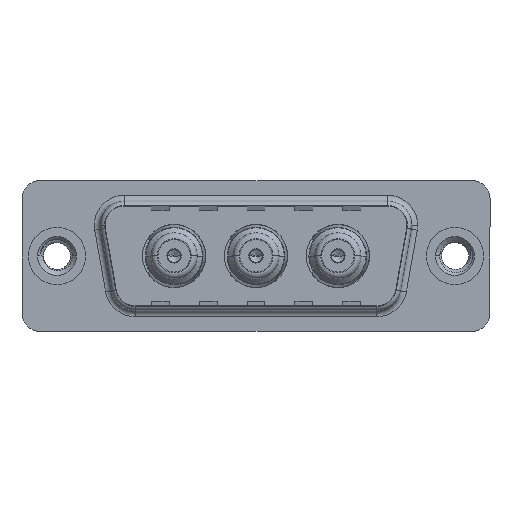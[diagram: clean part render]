
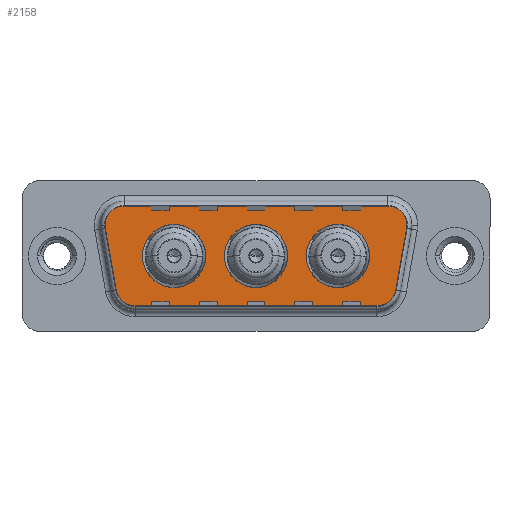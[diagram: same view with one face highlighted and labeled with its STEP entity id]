
A CAD part, top view. The second image highlights one B-rep face of the part: STEP entity #2158.
In plain terms, the highlighted planar face has unit normal (0, 0, 1).
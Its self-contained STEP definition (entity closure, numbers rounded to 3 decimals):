
#181 = CIRCLE ( 'NONE', #14283, 2.65 ) ;
#232 = DIRECTION ( 'NONE',  ( 1., 0., 0. ) ) ;
#323 = CARTESIAN_POINT ( 'NONE',  ( 3.441, 2.553, 0. ) ) ;
#436 = EDGE_LOOP ( 'NONE', ( #1682, #2005 ) ) ;
#500 = EDGE_CURVE ( 'NONE', #17174, #4676, #1837, .T. ) ;
#673 = CARTESIAN_POINT ( 'NONE',  ( 28.836, -3.247, 0. ) ) ;
#916 = DIRECTION ( 'NONE',  ( 1., 0., 0. ) ) ;
#1031 = VERTEX_POINT ( 'NONE', #10401 ) ;
#1154 = AXIS2_PLACEMENT_3D ( 'NONE', #15746, #4045, #232 ) ;
#1682 = ORIENTED_EDGE ( 'NONE', *, *, #6359, .F. ) ;
#1809 = PLANE ( 'NONE',  #12351 ) ;
#1837 = LINE ( 'NONE', #5329, #13462 ) ;
#1903 = CIRCLE ( 'NONE', #2619, 2.65 ) ;
#1958 = DIRECTION ( 'NONE',  ( 1., 0., 0. ) ) ;
#2002 = AXIS2_PLACEMENT_3D ( 'NONE', #4181, #14785, #5699 ) ;
#2005 = ORIENTED_EDGE ( 'NONE', *, *, #2195, .F. ) ;
#2093 = DIRECTION ( 'NONE',  ( -1., 0., 0. ) ) ;
#2158 = ADVANCED_FACE ( 'NONE', ( #16734, #5149, #18129, #12742 ), #1809, .T. ) ;
#2195 = EDGE_CURVE ( 'NONE', #3251, #8735, #4196, .T. ) ;
#2500 = VERTEX_POINT ( 'NONE', #8867 ) ;
#2619 = AXIS2_PLACEMENT_3D ( 'NONE', #13591, #13808, #13867 ) ;
#2841 = DIRECTION ( 'NONE',  ( 1., 0., 0. ) ) ;
#2946 = EDGE_CURVE ( 'NONE', #10367, #4493, #3212, .T. ) ;
#3025 = CARTESIAN_POINT ( 'NONE',  ( 16.65, 0., 0. ) ) ;
#3212 = CIRCLE ( 'NONE', #7172, 2.65 ) ;
#3251 = VERTEX_POINT ( 'NONE', #14914 ) ;
#3342 = CIRCLE ( 'NONE', #14150, 2. ) ;
#3473 = EDGE_CURVE ( 'NONE', #14745, #5964, #15758, .T. ) ;
#3595 = EDGE_CURVE ( 'NONE', #9859, #11575, #17843, .T. ) ;
#3685 = VECTOR ( 'NONE', #16691, 1000. ) ;
#3847 = AXIS2_PLACEMENT_3D ( 'NONE', #8420, #18898, #9929 ) ;
#4045 = DIRECTION ( 'NONE',  ( 0., 0., 1. ) ) ;
#4118 = CARTESIAN_POINT ( 'NONE',  ( 26.866, -4.9, 0. ) ) ;
#4178 = CIRCLE ( 'NONE', #9466, 2. ) ;
#4181 = CARTESIAN_POINT ( 'NONE',  ( 5.411, 2.9, 0. ) ) ;
#4196 = CIRCLE ( 'NONE', #14377, 2.65 ) ;
#4300 = DIRECTION ( 'NONE',  ( 0.174, 0.985, 0. ) ) ;
#4339 = CARTESIAN_POINT ( 'NONE',  ( 6.434, -4.9, 0. ) ) ;
#4355 = EDGE_CURVE ( 'NONE', #4493, #10367, #15504, .T. ) ;
#4493 = VERTEX_POINT ( 'NONE', #9935 ) ;
#4676 = VERTEX_POINT ( 'NONE', #7659 ) ;
#4897 = VERTEX_POINT ( 'NONE', #4118 ) ;
#4936 = VECTOR ( 'NONE', #1958, 1000. ) ;
#5143 = ORIENTED_EDGE ( 'NONE', *, *, #4355, .F. ) ;
#5149 = FACE_BOUND ( 'NONE', #9118, .T. ) ;
#5166 = CARTESIAN_POINT ( 'NONE',  ( 19.3, 0., 0. ) ) ;
#5329 = CARTESIAN_POINT ( 'NONE',  ( 3.441, 2.553, 0. ) ) ;
#5501 = EDGE_CURVE ( 'NONE', #10274, #1031, #181, .T. ) ;
#5699 = DIRECTION ( 'NONE',  ( 1., 0., 0. ) ) ;
#5873 = ORIENTED_EDGE ( 'NONE', *, *, #500, .T. ) ;
#5964 = VERTEX_POINT ( 'NONE', #9702 ) ;
#6044 = ORIENTED_EDGE ( 'NONE', *, *, #2946, .F. ) ;
#6244 = EDGE_CURVE ( 'NONE', #2500, #14745, #3342, .T. ) ;
#6270 = EDGE_CURVE ( 'NONE', #4676, #15197, #6930, .T. ) ;
#6359 = EDGE_CURVE ( 'NONE', #8735, #3251, #1903, .T. ) ;
#6642 = ORIENTED_EDGE ( 'NONE', *, *, #3473, .T. ) ;
#6729 = ORIENTED_EDGE ( 'NONE', *, *, #6270, .T. ) ;
#6782 = DIRECTION ( 'NONE',  ( 0., 0., 1. ) ) ;
#6930 = CIRCLE ( 'NONE', #17194, 2. ) ;
#7172 = AXIS2_PLACEMENT_3D ( 'NONE', #9135, #16872, #12388 ) ;
#7367 = EDGE_LOOP ( 'NONE', ( #11628, #17255, #19658, #19145, #6642, #17421, #5873, #6729, #8833 ) ) ;
#7417 = CARTESIAN_POINT ( 'NONE',  ( 26.866, -2.9, 0. ) ) ;
#7509 = EDGE_LOOP ( 'NONE', ( #9656, #10032 ) ) ;
#7659 = CARTESIAN_POINT ( 'NONE',  ( 4.464, -3.247, 0. ) ) ;
#8420 = CARTESIAN_POINT ( 'NONE',  ( 27.889, 2.9, 0. ) ) ;
#8735 = VERTEX_POINT ( 'NONE', #5166 ) ;
#8801 = DIRECTION ( 'NONE',  ( 0.174, -0.985, 0. ) ) ;
#8833 = ORIENTED_EDGE ( 'NONE', *, *, #10405, .T. ) ;
#8867 = CARTESIAN_POINT ( 'NONE',  ( 29.889, 2.9, 0. ) ) ;
#8975 = DIRECTION ( 'NONE',  ( 1., 0., 0. ) ) ;
#8986 = DIRECTION ( 'NONE',  ( 1., 0., 0. ) ) ;
#9118 = EDGE_LOOP ( 'NONE', ( #5143, #6044 ) ) ;
#9135 = CARTESIAN_POINT ( 'NONE',  ( 23.5, 0., 0. ) ) ;
#9379 = DIRECTION ( 'NONE',  ( 0., 0., 1. ) ) ;
#9466 = AXIS2_PLACEMENT_3D ( 'NONE', #7417, #17929, #8975 ) ;
#9528 = LINE ( 'NONE', #11101, #4936 ) ;
#9656 = ORIENTED_EDGE ( 'NONE', *, *, #5501, .F. ) ;
#9702 = CARTESIAN_POINT ( 'NONE',  ( 5.411, 4.9, 0. ) ) ;
#9719 = CARTESIAN_POINT ( 'NONE',  ( 6.434, -2.9, 0. ) ) ;
#9859 = VERTEX_POINT ( 'NONE', #673 ) ;
#9929 = DIRECTION ( 'NONE',  ( -1., 0., 0. ) ) ;
#9935 = CARTESIAN_POINT ( 'NONE',  ( 26.15, 0., 0. ) ) ;
#10032 = ORIENTED_EDGE ( 'NONE', *, *, #15024, .F. ) ;
#10105 = DIRECTION ( 'NONE',  ( 0., 0., 1. ) ) ;
#10181 = CIRCLE ( 'NONE', #2002, 2. ) ;
#10274 = VERTEX_POINT ( 'NONE', #15232 ) ;
#10367 = VERTEX_POINT ( 'NONE', #16999 ) ;
#10401 = CARTESIAN_POINT ( 'NONE',  ( 7.15, 0., 0. ) ) ;
#10405 = EDGE_CURVE ( 'NONE', #15197, #4897, #9528, .T. ) ;
#11101 = CARTESIAN_POINT ( 'NONE',  ( 6.434, -4.9, 0. ) ) ;
#11575 = VERTEX_POINT ( 'NONE', #15520 ) ;
#11628 = ORIENTED_EDGE ( 'NONE', *, *, #12701, .T. ) ;
#11911 = EDGE_CURVE ( 'NONE', #5964, #17174, #10181, .T. ) ;
#12206 = CARTESIAN_POINT ( 'NONE',  ( 29.859, 2.553, 0. ) ) ;
#12351 = AXIS2_PLACEMENT_3D ( 'NONE', #18287, #9379, #8986 ) ;
#12388 = DIRECTION ( 'NONE',  ( 1., 0., 0. ) ) ;
#12701 = EDGE_CURVE ( 'NONE', #4897, #9859, #4178, .T. ) ;
#12742 = FACE_OUTER_BOUND ( 'NONE', #7367, .T. ) ;
#13361 = DIRECTION ( 'NONE',  ( 0., 0., 1. ) ) ;
#13462 = VECTOR ( 'NONE', #8801, 1000. ) ;
#13591 = CARTESIAN_POINT ( 'NONE',  ( 16.65, 0., 0. ) ) ;
#13601 = CIRCLE ( 'NONE', #3847, 2. ) ;
#13808 = DIRECTION ( 'NONE',  ( 0., 0., 1. ) ) ;
#13829 = CIRCLE ( 'NONE', #15512, 2.65 ) ;
#13867 = DIRECTION ( 'NONE',  ( 1., 0., 0. ) ) ;
#14150 = AXIS2_PLACEMENT_3D ( 'NONE', #15932, #15672, #15605 ) ;
#14283 = AXIS2_PLACEMENT_3D ( 'NONE', #15786, #15696, #19221 ) ;
#14377 = AXIS2_PLACEMENT_3D ( 'NONE', #3025, #6782, #2841 ) ;
#14745 = VERTEX_POINT ( 'NONE', #18225 ) ;
#14785 = DIRECTION ( 'NONE',  ( 0., 0., 1. ) ) ;
#14914 = CARTESIAN_POINT ( 'NONE',  ( 14., 0., 0. ) ) ;
#15024 = EDGE_CURVE ( 'NONE', #1031, #10274, #13829, .T. ) ;
#15197 = VERTEX_POINT ( 'NONE', #4339 ) ;
#15232 = CARTESIAN_POINT ( 'NONE',  ( 12.45, 0., 0. ) ) ;
#15504 = CIRCLE ( 'NONE', #1154, 2.65 ) ;
#15512 = AXIS2_PLACEMENT_3D ( 'NONE', #19063, #10105, #916 ) ;
#15520 = CARTESIAN_POINT ( 'NONE',  ( 29.859, 2.553, 0. ) ) ;
#15605 = DIRECTION ( 'NONE',  ( -1., 0., 0. ) ) ;
#15672 = DIRECTION ( 'NONE',  ( 0., 0., 1. ) ) ;
#15696 = DIRECTION ( 'NONE',  ( 0., 0., 1. ) ) ;
#15746 = CARTESIAN_POINT ( 'NONE',  ( 23.5, 0., 0. ) ) ;
#15758 = LINE ( 'NONE', #17548, #3685 ) ;
#15786 = CARTESIAN_POINT ( 'NONE',  ( 9.8, 0., 0. ) ) ;
#15863 = EDGE_CURVE ( 'NONE', #11575, #2500, #13601, .T. ) ;
#15932 = CARTESIAN_POINT ( 'NONE',  ( 27.889, 2.9, 0. ) ) ;
#16691 = DIRECTION ( 'NONE',  ( -1., 0., 0. ) ) ;
#16734 = FACE_BOUND ( 'NONE', #436, .T. ) ;
#16872 = DIRECTION ( 'NONE',  ( 0., 0., 1. ) ) ;
#16999 = CARTESIAN_POINT ( 'NONE',  ( 20.85, 0., 0. ) ) ;
#17174 = VERTEX_POINT ( 'NONE', #323 ) ;
#17194 = AXIS2_PLACEMENT_3D ( 'NONE', #9719, #13361, #2093 ) ;
#17255 = ORIENTED_EDGE ( 'NONE', *, *, #3595, .T. ) ;
#17389 = VECTOR ( 'NONE', #4300, 1000. ) ;
#17421 = ORIENTED_EDGE ( 'NONE', *, *, #11911, .T. ) ;
#17548 = CARTESIAN_POINT ( 'NONE',  ( 5.411, 4.9, 0. ) ) ;
#17843 = LINE ( 'NONE', #12206, #17389 ) ;
#17929 = DIRECTION ( 'NONE',  ( 0., 0., 1. ) ) ;
#18129 = FACE_BOUND ( 'NONE', #7509, .T. ) ;
#18225 = CARTESIAN_POINT ( 'NONE',  ( 27.889, 4.9, 0. ) ) ;
#18287 = CARTESIAN_POINT ( 'NONE',  ( 26.866, -2.9, 0. ) ) ;
#18898 = DIRECTION ( 'NONE',  ( 0., 0., 1. ) ) ;
#19063 = CARTESIAN_POINT ( 'NONE',  ( 9.8, 0., 0. ) ) ;
#19145 = ORIENTED_EDGE ( 'NONE', *, *, #6244, .T. ) ;
#19221 = DIRECTION ( 'NONE',  ( 1., 0., 0. ) ) ;
#19658 = ORIENTED_EDGE ( 'NONE', *, *, #15863, .T. ) ;
